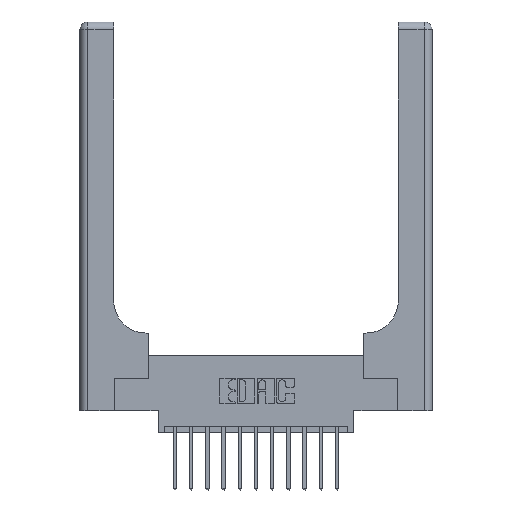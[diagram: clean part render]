
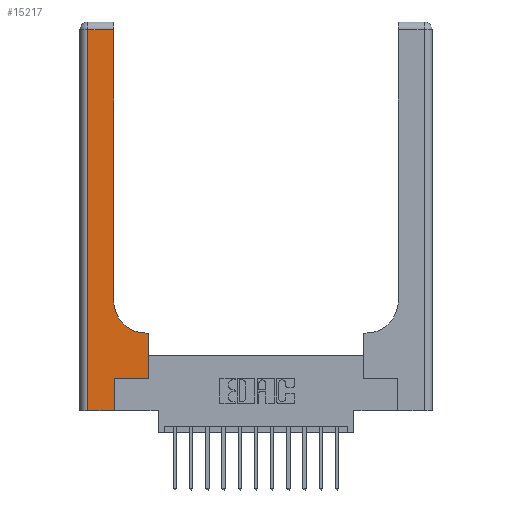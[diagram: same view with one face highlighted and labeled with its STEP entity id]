
A CAD part, top view. The second image highlights one B-rep face of the part: STEP entity #15217.
In plain terms, the highlighted planar face has unit normal (0, 0, 1).
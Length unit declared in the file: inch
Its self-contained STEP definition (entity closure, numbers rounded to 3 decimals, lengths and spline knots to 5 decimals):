
#554 = FACE_OUTER_BOUND ( 'NONE', #4702, .T. ) ;
#581 = CIRCLE ( 'NONE', #16351, 0.25 ) ;
#605 = CARTESIAN_POINT ( 'NONE',  ( 0.265, 0., 0.37 ) ) ;
#752 = CARTESIAN_POINT ( 'NONE',  ( 0.06, 2.94, 0.37 ) ) ;
#1737 = VECTOR ( 'NONE', #16487, 39.37008 ) ;
#1803 = EDGE_CURVE ( 'NONE', #12282, #16027, #9851, .T. ) ;
#2023 = EDGE_CURVE ( 'NONE', #11993, #12282, #15867, .T. ) ;
#2269 = VECTOR ( 'NONE', #3961, 39.37008 ) ;
#2363 = VERTEX_POINT ( 'NONE', #6854 ) ;
#2399 = LINE ( 'NONE', #16089, #9416 ) ;
#2569 = LINE ( 'NONE', #12337, #6647 ) ;
#2696 = EDGE_CURVE ( 'NONE', #7734, #6674, #11279, .T. ) ;
#2935 = DIRECTION ( 'NONE',  ( -1., 0., 0. ) ) ;
#3049 = CARTESIAN_POINT ( 'NONE',  ( 0.26, 3., 0.37 ) ) ;
#3087 = EDGE_CURVE ( 'NONE', #2363, #11993, #2399, .T. ) ;
#3229 = ORIENTED_EDGE ( 'NONE', *, *, #8138, .T. ) ;
#3764 = ORIENTED_EDGE ( 'NONE', *, *, #12911, .T. ) ;
#3871 = LINE ( 'NONE', #14652, #2269 ) ;
#3961 = DIRECTION ( 'NONE',  ( 1., 0., 0. ) ) ;
#3982 = EDGE_CURVE ( 'NONE', #14222, #7734, #2569, .T. ) ;
#4136 = ORIENTED_EDGE ( 'NONE', *, *, #1803, .T. ) ;
#4411 = DIRECTION ( 'NONE',  ( -1., 0., 0. ) ) ;
#4702 = EDGE_LOOP ( 'NONE', ( #3764, #8293, #16169, #4136, #8439, #8761, #6063, #16556, #3229 ) ) ;
#4863 = DIRECTION ( 'NONE',  ( -1., 0., 0. ) ) ;
#5630 = DIRECTION ( 'NONE',  ( 0., 1., 0. ) ) ;
#6063 = ORIENTED_EDGE ( 'NONE', *, *, #3982, .T. ) ;
#6647 = VECTOR ( 'NONE', #5630, 39.37008 ) ;
#6674 = VERTEX_POINT ( 'NONE', #7732 ) ;
#6854 = CARTESIAN_POINT ( 'NONE',  ( 0.26, 2.94, 0.37 ) ) ;
#7066 = VECTOR ( 'NONE', #8511, 39.37008 ) ;
#7199 = DIRECTION ( 'NONE',  ( 0., 0., -1. ) ) ;
#7239 = CARTESIAN_POINT ( 'NONE',  ( 0.51, 0.85, 0.37 ) ) ;
#7616 = CARTESIAN_POINT ( 'NONE',  ( 0.06, 3., 0.37 ) ) ;
#7732 = CARTESIAN_POINT ( 'NONE',  ( 0.51, 0.6, 0.37 ) ) ;
#7734 = VERTEX_POINT ( 'NONE', #15136 ) ;
#8138 = EDGE_CURVE ( 'NONE', #6674, #11656, #581, .T. ) ;
#8293 = ORIENTED_EDGE ( 'NONE', *, *, #3087, .T. ) ;
#8329 = LINE ( 'NONE', #15058, #7066 ) ;
#8439 = ORIENTED_EDGE ( 'NONE', *, *, #11029, .T. ) ;
#8511 = DIRECTION ( 'NONE',  ( 0., 1., 0. ) ) ;
#8539 = DIRECTION ( 'NONE',  ( 0., 0., -1. ) ) ;
#8569 = PLANE ( 'NONE',  #16078 ) ;
#8761 = ORIENTED_EDGE ( 'NONE', *, *, #9013, .T. ) ;
#8777 = DIRECTION ( 'NONE',  ( 1., 0., 0. ) ) ;
#8889 = CARTESIAN_POINT ( 'NONE',  ( 0., 0., 0.37 ) ) ;
#9013 = EDGE_CURVE ( 'NONE', #16106, #14222, #3871, .T. ) ;
#9120 = CARTESIAN_POINT ( 'NONE',  ( 0.26, 0.85, 0.37 ) ) ;
#9416 = VECTOR ( 'NONE', #2935, 39.37008 ) ;
#9690 = VECTOR ( 'NONE', #10751, 39.37008 ) ;
#9851 = LINE ( 'NONE', #8889, #1737 ) ;
#10751 = DIRECTION ( 'NONE',  ( 0., 1., 0. ) ) ;
#11029 = EDGE_CURVE ( 'NONE', #16027, #16106, #8329, .T. ) ;
#11189 = VECTOR ( 'NONE', #4411, 39.37008 ) ;
#11212 = CARTESIAN_POINT ( 'NONE',  ( 0., 3., 0.37 ) ) ;
#11279 = LINE ( 'NONE', #12410, #11189 ) ;
#11535 = CARTESIAN_POINT ( 'NONE',  ( 0.265, 0.25, 0.37 ) ) ;
#11656 = VERTEX_POINT ( 'NONE', #9120 ) ;
#11993 = VERTEX_POINT ( 'NONE', #752 ) ;
#12282 = VERTEX_POINT ( 'NONE', #12371 ) ;
#12337 = CARTESIAN_POINT ( 'NONE',  ( 0.528, 0.25, 0.37 ) ) ;
#12371 = CARTESIAN_POINT ( 'NONE',  ( 0.06, 0., 0.37 ) ) ;
#12389 = LINE ( 'NONE', #3049, #9690 ) ;
#12410 = CARTESIAN_POINT ( 'NONE',  ( 0.26, 0.6, 0.37 ) ) ;
#12548 = VECTOR ( 'NONE', #15302, 39.37008 ) ;
#12911 = EDGE_CURVE ( 'NONE', #11656, #2363, #12389, .T. ) ;
#14222 = VERTEX_POINT ( 'NONE', #14850 ) ;
#14652 = CARTESIAN_POINT ( 'NONE',  ( 0.265, 0.25, 0.37 ) ) ;
#14850 = CARTESIAN_POINT ( 'NONE',  ( 0.528, 0.25, 0.37 ) ) ;
#15058 = CARTESIAN_POINT ( 'NONE',  ( 0.265, 0., 0.37 ) ) ;
#15136 = CARTESIAN_POINT ( 'NONE',  ( 0.528, 0.6, 0.37 ) ) ;
#15217 = ADVANCED_FACE ( 'NONE', ( #554 ), #8569, .F. ) ;
#15302 = DIRECTION ( 'NONE',  ( 0., -1., 0. ) ) ;
#15867 = LINE ( 'NONE', #7616, #12548 ) ;
#16027 = VERTEX_POINT ( 'NONE', #605 ) ;
#16078 = AXIS2_PLACEMENT_3D ( 'NONE', #11212, #7199, #4863 ) ;
#16089 = CARTESIAN_POINT ( 'NONE',  ( 0., 2.94, 0.37 ) ) ;
#16106 = VERTEX_POINT ( 'NONE', #11535 ) ;
#16169 = ORIENTED_EDGE ( 'NONE', *, *, #2023, .T. ) ;
#16351 = AXIS2_PLACEMENT_3D ( 'NONE', #7239, #8539, #8777 ) ;
#16487 = DIRECTION ( 'NONE',  ( 1., 0., 0. ) ) ;
#16556 = ORIENTED_EDGE ( 'NONE', *, *, #2696, .T. ) ;
